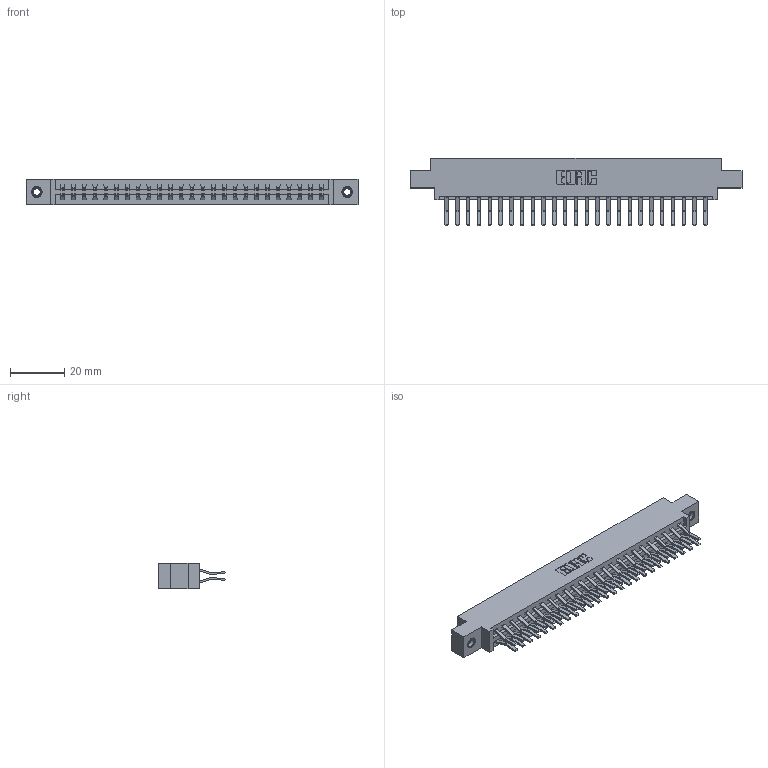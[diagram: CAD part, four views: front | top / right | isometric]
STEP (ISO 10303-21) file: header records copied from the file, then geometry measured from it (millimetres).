
FILE_DESCRIPTION (( 'STEP AP203' ), '1' );
FILE_NAME ('387-050-560-807.STEP', '2019-10-19T02:40:49', ( '' ), ( '' ), 'SwSTEP 2.0', 'SolidWorks 2016', '' );
FILE_SCHEMA (( 'CONFIG_CONTROL_DESIGN' ));
Length unit declared in the file: inch
Products named in the file (4): 387-050-560-807; 345-250-001_345-250-005-103; 345-292-001_560 Tail; 337 Part_0.170 Offset - 0.156 Dia-TI
Assembly tree (53 placements, depth 2):
  387-050-560-807
    337 Part_0.170 Offset - 0.156 Dia-TI
    345-292-001_560 Tail  x50
    345-250-001_345-250-005-103  x2
Bounding box: 122.07 x 24.78 x 9.4 mm (x, y, z)
Volume: 12835.4 mm3; surface area: 15437.6 mm2
Topology: 53 solids, 53 shells, 2978 faces, 8809 edges, 5798 vertices
Faces by surface type: plane 2006, cylinder 956, cone 12, torus 4
Entity records: 22988 total; most frequent: CARTESIAN_POINT 3869, ORIENTED_EDGE 3798, DIRECTION 3357, EDGE_CURVE 1899, VECTOR 1747, LINE 1747, VERTEX_POINT 1260, AXIS2_PLACEMENT_3D 805
